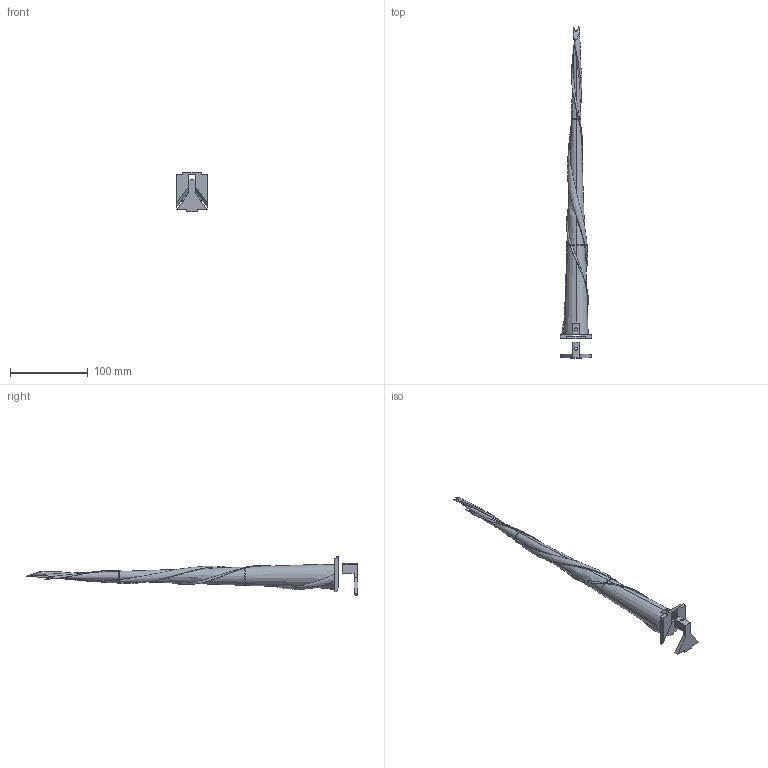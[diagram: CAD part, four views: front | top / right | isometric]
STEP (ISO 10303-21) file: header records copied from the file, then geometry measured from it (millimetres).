
FILE_DESCRIPTION (( 'STEP AP214' ), '1' );
FILE_NAME ('NarwhalNVG.STEP', '2020-05-01T17:25:21', ( '' ), ( '' ), 'SwSTEP 2.0', 'SolidWorks 2019', '' );
FILE_SCHEMA (( 'AUTOMOTIVE_DESIGN' ));
Length unit declared in the file: millimetre
Products named in the file (1): NarwhalNVG
Bounding box: 41 x 427.5 x 51.5 mm (x, y, z)
Volume: 128670.7 mm3; surface area: 36239.8 mm2
Topology: 4 solids, 4 shells, 91 faces, 254 edges, 167 vertices
Faces by surface type: plane 49, cone 18, bspline 15, cylinder 9
Entity records: 11110 total; most frequent: CARTESIAN_POINT 8926, ORIENTED_EDGE 508, DIRECTION 353, EDGE_CURVE 254, VERTEX_POINT 167, LINE 129, VECTOR 129, AXIS2_PLACEMENT_3D 112
